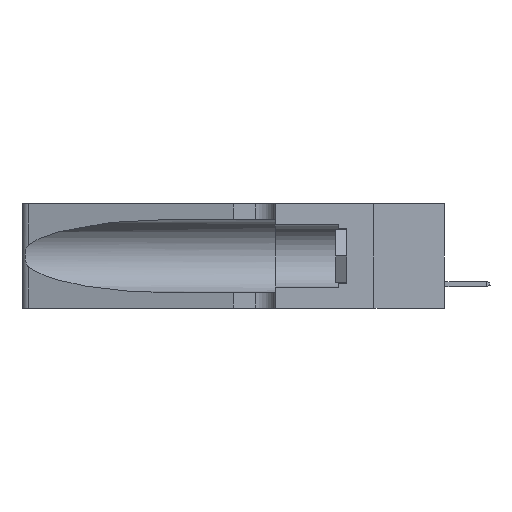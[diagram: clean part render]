
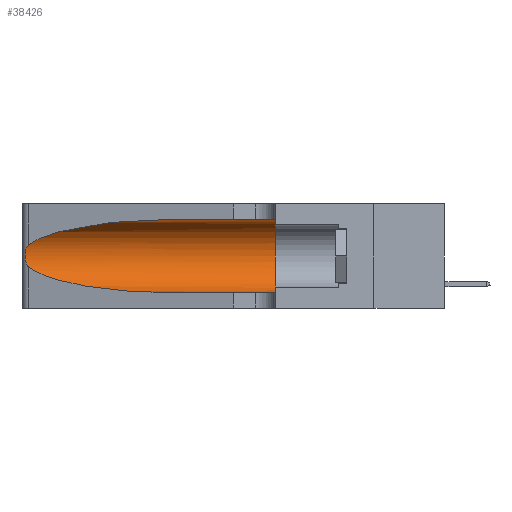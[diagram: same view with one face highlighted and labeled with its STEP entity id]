
A CAD part, left-side view. The second image highlights one B-rep face of the part: STEP entity #38426.
In plain terms, the highlighted cylindrical face has radius 3.308 mm (diameter 6.617 mm), a partial arc.
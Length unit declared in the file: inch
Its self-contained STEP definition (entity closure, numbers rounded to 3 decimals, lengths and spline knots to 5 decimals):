
#316 = LINE ( 'NONE', #3731, #26953 ) ;
#722 = CARTESIAN_POINT ( 'NONE',  ( 0.26075, 1.23896, 0.178 ) ) ;
#830 = EDGE_CURVE ( 'NONE', #988, #44131, #33115, .T. ) ;
#988 = VERTEX_POINT ( 'NONE', #13777 ) ;
#2584 = FACE_OUTER_BOUND ( 'NONE', #21259, .T. ) ;
#2827 = VERTEX_POINT ( 'NONE', #14471 ) ;
#3630 = CARTESIAN_POINT ( 'NONE',  ( 0.1305, 0.72297, 0.05475 ) ) ;
#3731 = CARTESIAN_POINT ( 'NONE',  ( 0.1305, 1.61858, 0.31525 ) ) ;
#4114 = DIRECTION ( 'NONE',  ( 0., 0., 1. ) ) ;
#5500 = VERTEX_POINT ( 'NONE', #36690 ) ;
#5513 = CARTESIAN_POINT ( 'NONE',  ( 0.18966, 0.96281, 0.05475 ) ) ;
#6534 = EDGE_CURVE ( 'NONE', #5500, #43522, #6723, .T. ) ;
#6723 =( BOUNDED_CURVE ( )  B_SPLINE_CURVE ( 3, ( #35544, #42280, #28108, #17519 ),
 .UNSPECIFIED., .F., .T. ) 
 B_SPLINE_CURVE_WITH_KNOTS ( ( 4, 4 ),
 ( 1.5708, 2.84003 ),
 .UNSPECIFIED. ) 
 CURVE ( )  GEOMETRIC_REPRESENTATION_ITEM ( )  RATIONAL_B_SPLINE_CURVE ( ( 1., 0.87, 0.87, 1. ) ) 
 REPRESENTATION_ITEM ( '' )  );
#8927 = DIRECTION ( 'NONE',  ( 0., 0., -1. ) ) ;
#9407 = CYLINDRICAL_SURFACE ( 'NONE', #38480, 0.13025 ) ;
#10792 = ORIENTED_EDGE ( 'NONE', *, *, #40547, .T. ) ;
#11238 = CARTESIAN_POINT ( 'NONE',  ( 0.25639, 1.23184, 0.21858 ) ) ;
#11969 = AXIS2_PLACEMENT_3D ( 'NONE', #36287, #29179, #4114 ) ;
#11993 = CARTESIAN_POINT ( 'NONE',  ( 0.25487, 1.22718, 0.14631 ) ) ;
#13232 = DIRECTION ( 'NONE',  ( 0., -1., 0. ) ) ;
#13777 = CARTESIAN_POINT ( 'NONE',  ( 0.25487, 1.22718, 0.14631 ) ) ;
#14470 = CARTESIAN_POINT ( 'NONE',  ( 0.25487, 1.22718, 0.22369 ) ) ;
#14471 = CARTESIAN_POINT ( 'NONE',  ( 0.1305, 0.35, 0.31525 ) ) ;
#15177 = CARTESIAN_POINT ( 'NONE',  ( 0.25639, 1.23186, 0.15144 ) ) ;
#16465 = CARTESIAN_POINT ( 'NONE',  ( 0.2373, 1.15595, 0.08982 ) ) ;
#16713 = CARTESIAN_POINT ( 'NONE',  ( 0.1305, 1.61858, 0.185 ) ) ;
#17519 = CARTESIAN_POINT ( 'NONE',  ( 0.25487, 1.22718, 0.22369 ) ) ;
#18273 = CARTESIAN_POINT ( 'NONE',  ( 0.25854, 1.2359, 0.20912 ) ) ;
#19430 = CIRCLE ( 'NONE', #11969, 0.13025 ) ;
#20295 = EDGE_CURVE ( 'NONE', #5500, #2827, #316, .T. ) ;
#21259 = EDGE_LOOP ( 'NONE', ( #27145, #34617, #27000, #10792, #29078, #41934 ) ) ;
#22217 = DIRECTION ( 'NONE',  ( 0., -1., 0. ) ) ;
#22931 = CARTESIAN_POINT ( 'NONE',  ( 0.26017, 1.23833, 0.17102 ) ) ;
#25504 = CARTESIAN_POINT ( 'NONE',  ( 0.26018, 1.23835, 0.19895 ) ) ;
#26953 = VECTOR ( 'NONE', #22217, 39.37008 ) ;
#26980 = CARTESIAN_POINT ( 'NONE',  ( 0.1305, 0.35, 0.05475 ) ) ;
#27000 = ORIENTED_EDGE ( 'NONE', *, *, #830, .T. ) ;
#27145 = ORIENTED_EDGE ( 'NONE', *, *, #6534, .T. ) ;
#27204 = CARTESIAN_POINT ( 'NONE',  ( 0.25487, 1.22718, 0.14631 ) ) ;
#27377 = CARTESIAN_POINT ( 'NONE',  ( 0.1305, 0.72297, 0.05475 ) ) ;
#27688 = CARTESIAN_POINT ( 'NONE',  ( 0.25487, 1.22718, 0.22369 ) ) ;
#27754 = VERTEX_POINT ( 'NONE', #26980 ) ;
#28108 = CARTESIAN_POINT ( 'NONE',  ( 0.2373, 1.15595, 0.28018 ) ) ;
#29078 = ORIENTED_EDGE ( 'NONE', *, *, #41671, .F. ) ;
#29179 = DIRECTION ( 'NONE',  ( 0., 1., 0. ) ) ;
#29279 = EDGE_CURVE ( 'NONE', #43522, #988, #29323, .T. ) ;
#29323 = B_SPLINE_CURVE_WITH_KNOTS ( 'NONE', 3,
 ( #27688, #39447, #11238, #39750, #18273, #25504, #29618, #722, #22931, #33684, #33226, #15177, #44567, #11993 ),
 .UNSPECIFIED., .F., .F.,
 ( 4, 2, 2, 2, 2, 2, 4 ),
 ( 0., 0.00027, 0.00053, 0.00107, 0.0016, 0.00187, 0.00214 ),
 .UNSPECIFIED. ) ;
#29618 = CARTESIAN_POINT ( 'NONE',  ( 0.26075, 1.23896, 0.19203 ) ) ;
#33115 =( BOUNDED_CURVE ( )  B_SPLINE_CURVE ( 3, ( #27204, #16465, #5513, #27377 ),
 .UNSPECIFIED., .F., .T. ) 
 B_SPLINE_CURVE_WITH_KNOTS ( ( 4, 4 ),
 ( 3.44316, 4.71239 ),
 .UNSPECIFIED. ) 
 CURVE ( )  GEOMETRIC_REPRESENTATION_ITEM ( )  RATIONAL_B_SPLINE_CURVE ( ( 1., 0.87, 0.87, 1. ) ) 
 REPRESENTATION_ITEM ( '' )  );
#33226 = CARTESIAN_POINT ( 'NONE',  ( 0.25789, 1.23486, 0.15765 ) ) ;
#33684 = CARTESIAN_POINT ( 'NONE',  ( 0.25856, 1.23593, 0.16098 ) ) ;
#34617 = ORIENTED_EDGE ( 'NONE', *, *, #29279, .T. ) ;
#35544 = CARTESIAN_POINT ( 'NONE',  ( 0.1305, 0.72297, 0.31525 ) ) ;
#36287 = CARTESIAN_POINT ( 'NONE',  ( 0.1305, 0.35, 0.185 ) ) ;
#36690 = CARTESIAN_POINT ( 'NONE',  ( 0.1305, 0.72297, 0.31525 ) ) ;
#37081 = LINE ( 'NONE', #38292, #41579 ) ;
#38292 = CARTESIAN_POINT ( 'NONE',  ( 0.1305, 1.61858, 0.05475 ) ) ;
#38426 = ADVANCED_FACE ( 'NONE', ( #2584 ), #9407, .F. ) ;
#38480 = AXIS2_PLACEMENT_3D ( 'NONE', #16713, #13232, #8927 ) ;
#39447 = CARTESIAN_POINT ( 'NONE',  ( 0.25555, 1.22994, 0.2215 ) ) ;
#39750 = CARTESIAN_POINT ( 'NONE',  ( 0.25787, 1.23484, 0.2124 ) ) ;
#40547 = EDGE_CURVE ( 'NONE', #44131, #27754, #37081, .T. ) ;
#41579 = VECTOR ( 'NONE', #42215, 39.37008 ) ;
#41671 = EDGE_CURVE ( 'NONE', #2827, #27754, #19430, .T. ) ;
#41934 = ORIENTED_EDGE ( 'NONE', *, *, #20295, .F. ) ;
#42215 = DIRECTION ( 'NONE',  ( 0., -1., 0. ) ) ;
#42280 = CARTESIAN_POINT ( 'NONE',  ( 0.18966, 0.96281, 0.31525 ) ) ;
#43522 = VERTEX_POINT ( 'NONE', #14470 ) ;
#44131 = VERTEX_POINT ( 'NONE', #3630 ) ;
#44567 = CARTESIAN_POINT ( 'NONE',  ( 0.25555, 1.22993, 0.14849 ) ) ;
